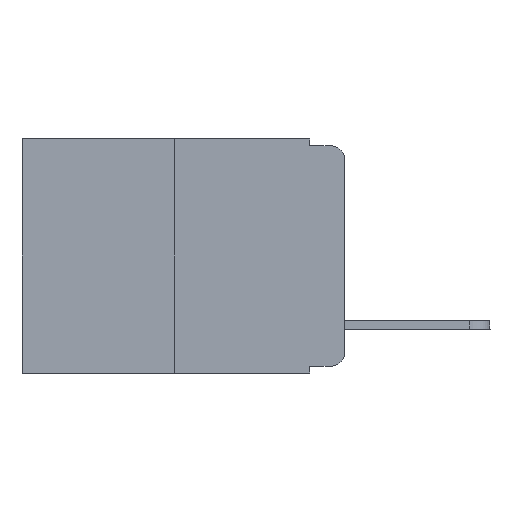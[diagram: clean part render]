
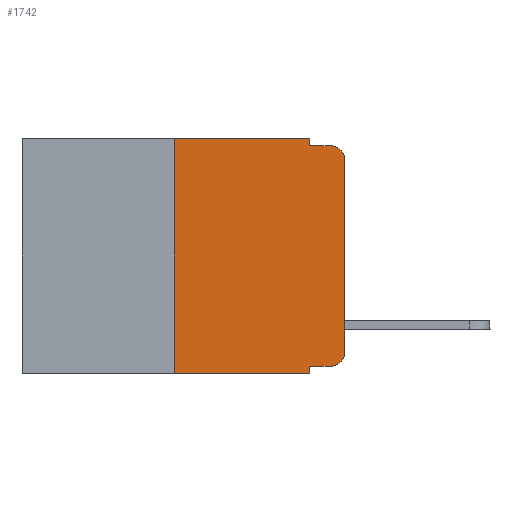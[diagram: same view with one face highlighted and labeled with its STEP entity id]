
A CAD part, left-side view. The second image highlights one B-rep face of the part: STEP entity #1742.
In plain terms, the highlighted planar face has unit normal (-1, 0, 0).
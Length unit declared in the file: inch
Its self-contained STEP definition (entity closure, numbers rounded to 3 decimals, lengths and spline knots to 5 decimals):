
#460 = VERTEX_POINT ( 'NONE', #3815 ) ;
#777 = CARTESIAN_POINT ( 'NONE',  ( 0., 0.051, 0. ) ) ;
#856 = DIRECTION ( 'NONE',  ( 0., 0., -1. ) ) ;
#1010 = VECTOR ( 'NONE', #16549, 39.37008 ) ;
#1188 = EDGE_CURVE ( 'NONE', #11114, #7967, #7039, .T. ) ;
#1586 = LINE ( 'NONE', #1693, #19459 ) ;
#1693 = CARTESIAN_POINT ( 'NONE',  ( 0., 0.051, -0.01 ) ) ;
#1742 = ADVANCED_FACE ( 'NONE', ( #4089 ), #11058, .F. ) ;
#2120 = EDGE_CURVE ( 'NONE', #7967, #14830, #2980, .T. ) ;
#2239 = LINE ( 'NONE', #777, #10678 ) ;
#2316 = AXIS2_PLACEMENT_3D ( 'NONE', #20127, #6226, #10617 ) ;
#2358 = DIRECTION ( 'NONE',  ( 0., -1., 0. ) ) ;
#2526 = EDGE_CURVE ( 'NONE', #14390, #9794, #2239, .T. ) ;
#2670 = EDGE_CURVE ( 'NONE', #9882, #14755, #10901, .T. ) ;
#2980 = CIRCLE ( 'NONE', #2316, 0.02 ) ;
#3173 = EDGE_CURVE ( 'NONE', #9794, #14830, #1586, .T. ) ;
#3815 = CARTESIAN_POINT ( 'NONE',  ( 0., 0.25, -0.343 ) ) ;
#3850 = LINE ( 'NONE', #8767, #4839 ) ;
#4014 = VECTOR ( 'NONE', #18839, 39.37008 ) ;
#4089 = FACE_OUTER_BOUND ( 'NONE', #13268, .T. ) ;
#4308 = ORIENTED_EDGE ( 'NONE', *, *, #16566, .T. ) ;
#4839 = VECTOR ( 'NONE', #11686, 39.37008 ) ;
#5049 = VECTOR ( 'NONE', #10805, 39.37008 ) ;
#5106 = ORIENTED_EDGE ( 'NONE', *, *, #1188, .T. ) ;
#5516 = CARTESIAN_POINT ( 'NONE',  ( 0., 0.051, -0.333 ) ) ;
#6226 = DIRECTION ( 'NONE',  ( -1., 0., 0. ) ) ;
#6481 = CARTESIAN_POINT ( 'NONE',  ( 0., 0.051, -0.01 ) ) ;
#6482 = DIRECTION ( 'NONE',  ( 0., -1., 0. ) ) ;
#6779 = DIRECTION ( 'NONE',  ( -1., 0., 0. ) ) ;
#7039 = LINE ( 'NONE', #18197, #1010 ) ;
#7361 = CARTESIAN_POINT ( 'NONE',  ( 0., 0.051, 0. ) ) ;
#7397 = CARTESIAN_POINT ( 'NONE',  ( 0., 0.051, -0.343 ) ) ;
#7788 = LINE ( 'NONE', #12778, #4014 ) ;
#7967 = VERTEX_POINT ( 'NONE', #15803 ) ;
#8000 = VERTEX_POINT ( 'NONE', #9031 ) ;
#8514 = EDGE_CURVE ( 'NONE', #16437, #14390, #15782, .T. ) ;
#8767 = CARTESIAN_POINT ( 'NONE',  ( 0., 0.25, 0. ) ) ;
#9031 = CARTESIAN_POINT ( 'NONE',  ( 0., 0.02, -0.333 ) ) ;
#9194 = CARTESIAN_POINT ( 'NONE',  ( 0., 0.473, 0. ) ) ;
#9794 = VERTEX_POINT ( 'NONE', #6481 ) ;
#9827 = CARTESIAN_POINT ( 'NONE',  ( 0., 0.473, 0. ) ) ;
#9838 = DIRECTION ( 'NONE',  ( 0., -1., 0. ) ) ;
#9882 = VERTEX_POINT ( 'NONE', #5516 ) ;
#10064 = CIRCLE ( 'NONE', #13055, 0.02 ) ;
#10617 = DIRECTION ( 'NONE',  ( 0., 0., -1. ) ) ;
#10678 = VECTOR ( 'NONE', #13489, 39.37008 ) ;
#10738 = CARTESIAN_POINT ( 'NONE',  ( 0., 0.02, -0.01 ) ) ;
#10805 = DIRECTION ( 'NONE',  ( 0., 0., -1. ) ) ;
#10901 = LINE ( 'NONE', #7361, #5049 ) ;
#11058 = PLANE ( 'NONE',  #13627 ) ;
#11111 = EDGE_CURVE ( 'NONE', #460, #16437, #3850, .T. ) ;
#11114 = VERTEX_POINT ( 'NONE', #19825 ) ;
#11602 = CARTESIAN_POINT ( 'NONE',  ( 0., 0.051, 0. ) ) ;
#11686 = DIRECTION ( 'NONE',  ( 0., 0., 1. ) ) ;
#11861 = ORIENTED_EDGE ( 'NONE', *, *, #8514, .F. ) ;
#12629 = VECTOR ( 'NONE', #6482, 39.37008 ) ;
#12778 = CARTESIAN_POINT ( 'NONE',  ( 0., 0.473, -0.343 ) ) ;
#13055 = AXIS2_PLACEMENT_3D ( 'NONE', #14586, #6779, #19300 ) ;
#13192 = ORIENTED_EDGE ( 'NONE', *, *, #17753, .T. ) ;
#13268 = EDGE_LOOP ( 'NONE', ( #5106, #18599, #14554, #18337, #11861, #13771, #4308, #18449, #14203, #13192 ) ) ;
#13443 = EDGE_CURVE ( 'NONE', #9882, #8000, #19691, .T. ) ;
#13489 = DIRECTION ( 'NONE',  ( 0., 0., -1. ) ) ;
#13627 = AXIS2_PLACEMENT_3D ( 'NONE', #9194, #18769, #856 ) ;
#13771 = ORIENTED_EDGE ( 'NONE', *, *, #11111, .F. ) ;
#14203 = ORIENTED_EDGE ( 'NONE', *, *, #13443, .T. ) ;
#14228 = VECTOR ( 'NONE', #2358, 39.37008 ) ;
#14390 = VERTEX_POINT ( 'NONE', #11602 ) ;
#14554 = ORIENTED_EDGE ( 'NONE', *, *, #3173, .F. ) ;
#14586 = CARTESIAN_POINT ( 'NONE',  ( 0., 0.02, -0.313 ) ) ;
#14755 = VERTEX_POINT ( 'NONE', #7397 ) ;
#14830 = VERTEX_POINT ( 'NONE', #10738 ) ;
#15782 = LINE ( 'NONE', #9827, #12629 ) ;
#15803 = CARTESIAN_POINT ( 'NONE',  ( 0., 0., -0.03 ) ) ;
#16437 = VERTEX_POINT ( 'NONE', #19898 ) ;
#16549 = DIRECTION ( 'NONE',  ( 0., 0., 1. ) ) ;
#16566 = EDGE_CURVE ( 'NONE', #460, #14755, #7788, .T. ) ;
#16664 = CARTESIAN_POINT ( 'NONE',  ( 0., 0.051, -0.333 ) ) ;
#17753 = EDGE_CURVE ( 'NONE', #8000, #11114, #10064, .T. ) ;
#18197 = CARTESIAN_POINT ( 'NONE',  ( 0., 0., 0. ) ) ;
#18337 = ORIENTED_EDGE ( 'NONE', *, *, #2526, .F. ) ;
#18449 = ORIENTED_EDGE ( 'NONE', *, *, #2670, .F. ) ;
#18599 = ORIENTED_EDGE ( 'NONE', *, *, #2120, .T. ) ;
#18769 = DIRECTION ( 'NONE',  ( 1., 0., 0. ) ) ;
#18839 = DIRECTION ( 'NONE',  ( 0., -1., 0. ) ) ;
#19300 = DIRECTION ( 'NONE',  ( 0., 0., -1. ) ) ;
#19459 = VECTOR ( 'NONE', #9838, 39.37008 ) ;
#19691 = LINE ( 'NONE', #16664, #14228 ) ;
#19825 = CARTESIAN_POINT ( 'NONE',  ( 0., 0., -0.313 ) ) ;
#19898 = CARTESIAN_POINT ( 'NONE',  ( 0., 0.25, 0. ) ) ;
#20127 = CARTESIAN_POINT ( 'NONE',  ( 0., 0.02, -0.03 ) ) ;
